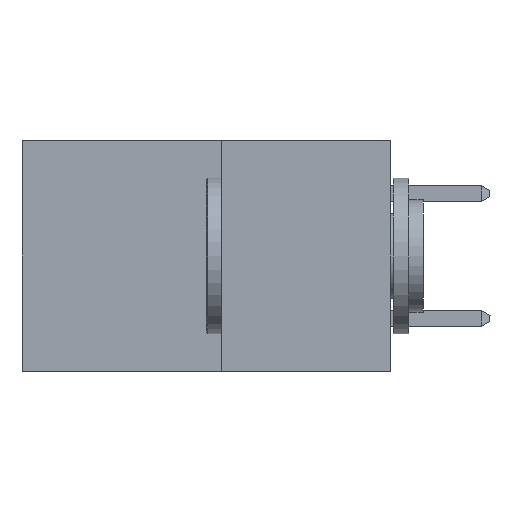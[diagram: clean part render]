
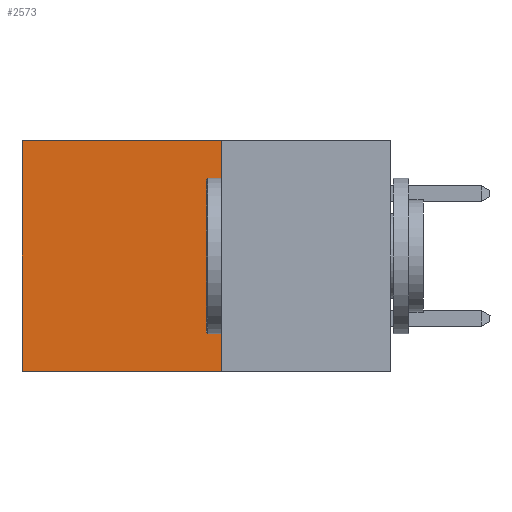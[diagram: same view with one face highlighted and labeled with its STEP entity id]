
A CAD part, left-side view. The second image highlights one B-rep face of the part: STEP entity #2573.
In plain terms, the highlighted planar face has unit normal (-1, 0, 0).
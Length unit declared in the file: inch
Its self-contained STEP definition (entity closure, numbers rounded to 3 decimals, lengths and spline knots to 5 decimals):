
#622 = EDGE_LOOP ( 'NONE', ( #8355, #9794, #7778, #9071 ) ) ;
#1702 = DIRECTION ( 'NONE',  ( 0., 0., -1. ) ) ;
#2338 = CARTESIAN_POINT ( 'NONE',  ( 0.277, 0.27, 0. ) ) ;
#2387 = LINE ( 'NONE', #6475, #10906 ) ;
#2407 = VECTOR ( 'NONE', #6033, 39.37008 ) ;
#2573 = ADVANCED_FACE ( 'NONE', ( #10961 ), #3782, .F. ) ;
#2712 = CARTESIAN_POINT ( 'NONE',  ( 0.277, 0.59, -0.37 ) ) ;
#2830 = VECTOR ( 'NONE', #1702, 39.37008 ) ;
#3136 = VERTEX_POINT ( 'NONE', #7515 ) ;
#3174 = CARTESIAN_POINT ( 'NONE',  ( 0.277, 0.27, -0.37 ) ) ;
#3300 = EDGE_CURVE ( 'NONE', #5080, #7034, #7172, .T. ) ;
#3642 = DIRECTION ( 'NONE',  ( 0., 0., -1. ) ) ;
#3681 = DIRECTION ( 'NONE',  ( 1., 0., 0. ) ) ;
#3782 = PLANE ( 'NONE',  #10786 ) ;
#3818 = CARTESIAN_POINT ( 'NONE',  ( 0.277, 0.27, -0.37 ) ) ;
#5080 = VERTEX_POINT ( 'NONE', #2338 ) ;
#5196 = CARTESIAN_POINT ( 'NONE',  ( 0.277, 0.27, 0. ) ) ;
#5576 = EDGE_CURVE ( 'NONE', #5080, #8019, #6501, .T. ) ;
#6033 = DIRECTION ( 'NONE',  ( 0., 1., 0. ) ) ;
#6202 = CARTESIAN_POINT ( 'NONE',  ( 0.277, 0.27, -0.37 ) ) ;
#6230 = EDGE_CURVE ( 'NONE', #8019, #3136, #9334, .T. ) ;
#6452 = EDGE_CURVE ( 'NONE', #7034, #3136, #2387, .T. ) ;
#6475 = CARTESIAN_POINT ( 'NONE',  ( 0.277, 0.27, -0.37 ) ) ;
#6501 = LINE ( 'NONE', #5196, #2407 ) ;
#6573 = DIRECTION ( 'NONE',  ( 0., 0., -1. ) ) ;
#6921 = VECTOR ( 'NONE', #6573, 39.37008 ) ;
#7034 = VERTEX_POINT ( 'NONE', #6202 ) ;
#7172 = LINE ( 'NONE', #3174, #6921 ) ;
#7508 = CARTESIAN_POINT ( 'NONE',  ( 0.277, 0.59, 0. ) ) ;
#7515 = CARTESIAN_POINT ( 'NONE',  ( 0.277, 0.59, -0.37 ) ) ;
#7778 = ORIENTED_EDGE ( 'NONE', *, *, #3300, .F. ) ;
#8019 = VERTEX_POINT ( 'NONE', #7508 ) ;
#8355 = ORIENTED_EDGE ( 'NONE', *, *, #6230, .T. ) ;
#9071 = ORIENTED_EDGE ( 'NONE', *, *, #5576, .T. ) ;
#9334 = LINE ( 'NONE', #2712, #2830 ) ;
#9794 = ORIENTED_EDGE ( 'NONE', *, *, #6452, .F. ) ;
#10786 = AXIS2_PLACEMENT_3D ( 'NONE', #3818, #3681, #3642 ) ;
#10906 = VECTOR ( 'NONE', #10921, 39.37008 ) ;
#10921 = DIRECTION ( 'NONE',  ( 0., 1., 0. ) ) ;
#10961 = FACE_OUTER_BOUND ( 'NONE', #622, .T. ) ;
